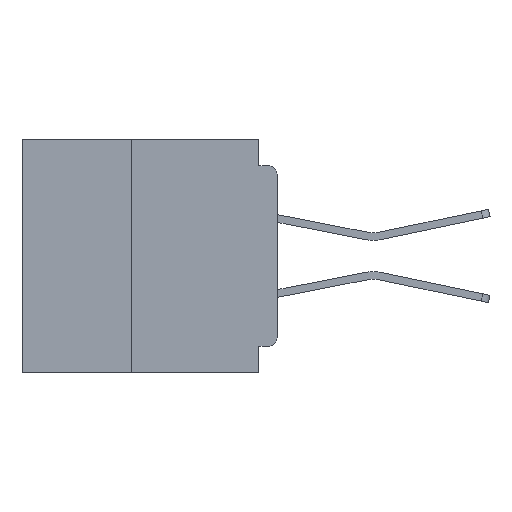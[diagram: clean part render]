
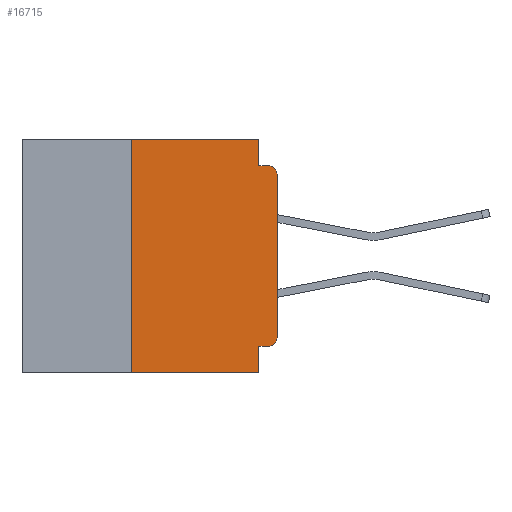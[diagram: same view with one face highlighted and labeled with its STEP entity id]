
A CAD part, left-side view. The second image highlights one B-rep face of the part: STEP entity #16715.
In plain terms, the highlighted planar face has unit normal (-1, 0, 0).
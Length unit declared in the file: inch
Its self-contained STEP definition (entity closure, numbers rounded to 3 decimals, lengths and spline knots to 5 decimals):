
#3455 = CARTESIAN_POINT ( 'NONE',  ( 0., 0., 0. ) ) ;
#4872 = CARTESIAN_POINT ( 'NONE',  ( 0., 0.015, -0.355 ) ) ;
#5386 = DIRECTION ( 'NONE',  ( 0., -1., 0. ) ) ;
#5834 = LINE ( 'NONE', #49728, #11250 ) ;
#6567 = CARTESIAN_POINT ( 'NONE',  ( 0., 0.437, -0.4 ) ) ;
#8471 = DIRECTION ( 'NONE',  ( 0., 0., 1. ) ) ;
#9504 = DIRECTION ( 'NONE',  ( -1., 0., 0. ) ) ;
#9772 = CARTESIAN_POINT ( 'NONE',  ( 0., 0.031, -0.355 ) ) ;
#10374 = EDGE_CURVE ( 'NONE', #25552, #42481, #11845, .T. ) ;
#10798 = DIRECTION ( 'NONE',  ( 0., -1., 0. ) ) ;
#11157 = DIRECTION ( 'NONE',  ( -1., 0., 0. ) ) ;
#11250 = VECTOR ( 'NONE', #5386, 39.37008 ) ;
#11527 = CARTESIAN_POINT ( 'NONE',  ( 0., 0.015, -0.045 ) ) ;
#11551 = DIRECTION ( 'NONE',  ( 0., -1., 0. ) ) ;
#11845 = LINE ( 'NONE', #53822, #62756 ) ;
#13513 = EDGE_CURVE ( 'NONE', #52806, #45331, #13784, .T. ) ;
#13784 = LINE ( 'NONE', #21870, #38605 ) ;
#14184 = LINE ( 'NONE', #3455, #48982 ) ;
#16715 = ADVANCED_FACE ( 'NONE', ( #23453 ), #50948, .F. ) ;
#17158 = CARTESIAN_POINT ( 'NONE',  ( 0., 0.25, 0. ) ) ;
#18208 = CARTESIAN_POINT ( 'NONE',  ( 0., 0.25, -0.4 ) ) ;
#18677 = VERTEX_POINT ( 'NONE', #47923 ) ;
#18728 = LINE ( 'NONE', #40527, #33499 ) ;
#19309 = LINE ( 'NONE', #6567, #44117 ) ;
#19491 = VERTEX_POINT ( 'NONE', #59799 ) ;
#19606 = ORIENTED_EDGE ( 'NONE', *, *, #21280, .F. ) ;
#21280 = EDGE_CURVE ( 'NONE', #45331, #45903, #18728, .T. ) ;
#21620 = AXIS2_PLACEMENT_3D ( 'NONE', #46044, #55880, #26408 ) ;
#21870 = CARTESIAN_POINT ( 'NONE',  ( 0., 0.031, 0. ) ) ;
#23093 = CARTESIAN_POINT ( 'NONE',  ( 0., 0.031, -0.4 ) ) ;
#23453 = FACE_OUTER_BOUND ( 'NONE', #51511, .T. ) ;
#23749 = ORIENTED_EDGE ( 'NONE', *, *, #13513, .F. ) ;
#25552 = VERTEX_POINT ( 'NONE', #4872 ) ;
#25715 = ORIENTED_EDGE ( 'NONE', *, *, #50048, .T. ) ;
#26408 = DIRECTION ( 'NONE',  ( 0., 0., -1. ) ) ;
#27443 = EDGE_CURVE ( 'NONE', #25552, #18677, #63389, .T. ) ;
#29066 = VERTEX_POINT ( 'NONE', #47183 ) ;
#29164 = EDGE_CURVE ( 'NONE', #29066, #30611, #31685, .T. ) ;
#30611 = VERTEX_POINT ( 'NONE', #17158 ) ;
#31685 = LINE ( 'NONE', #18208, #41741 ) ;
#31871 = DIRECTION ( 'NONE',  ( 0., 0., -1. ) ) ;
#33196 = DIRECTION ( 'NONE',  ( 0., 0., 1. ) ) ;
#33471 = VERTEX_POINT ( 'NONE', #23093 ) ;
#33499 = VECTOR ( 'NONE', #10798, 39.37008 ) ;
#33875 = EDGE_CURVE ( 'NONE', #29066, #33471, #19309, .T. ) ;
#35466 = VECTOR ( 'NONE', #45686, 39.37008 ) ;
#36401 = ORIENTED_EDGE ( 'NONE', *, *, #47522, .F. ) ;
#38605 = VECTOR ( 'NONE', #31871, 39.37008 ) ;
#39180 = ORIENTED_EDGE ( 'NONE', *, *, #46411, .F. ) ;
#39201 = CARTESIAN_POINT ( 'NONE',  ( 0., 0.015, -0.34 ) ) ;
#40527 = CARTESIAN_POINT ( 'NONE',  ( 0., 0., -0.045 ) ) ;
#40738 = CARTESIAN_POINT ( 'NONE',  ( 0., 0.031, -0.4 ) ) ;
#40873 = CARTESIAN_POINT ( 'NONE',  ( 0., 0.015, -0.06 ) ) ;
#41687 = LINE ( 'NONE', #40738, #35466 ) ;
#41741 = VECTOR ( 'NONE', #33196, 39.37008 ) ;
#42357 = ORIENTED_EDGE ( 'NONE', *, *, #29164, .F. ) ;
#42481 = VERTEX_POINT ( 'NONE', #9772 ) ;
#44117 = VECTOR ( 'NONE', #11551, 39.37008 ) ;
#44195 = DIRECTION ( 'NONE',  ( 0., 0., -1. ) ) ;
#44206 = DIRECTION ( 'NONE',  ( 0., 1., 0. ) ) ;
#45331 = VERTEX_POINT ( 'NONE', #56497 ) ;
#45686 = DIRECTION ( 'NONE',  ( 0., 0., -1. ) ) ;
#45816 = DIRECTION ( 'NONE',  ( 0., 0., -1. ) ) ;
#45903 = VERTEX_POINT ( 'NONE', #11527 ) ;
#46044 = CARTESIAN_POINT ( 'NONE',  ( 0., 0.437, 0. ) ) ;
#46411 = EDGE_CURVE ( 'NONE', #42481, #33471, #41687, .T. ) ;
#47183 = CARTESIAN_POINT ( 'NONE',  ( 0., 0.25, -0.4 ) ) ;
#47522 = EDGE_CURVE ( 'NONE', #30611, #52806, #5834, .T. ) ;
#47923 = CARTESIAN_POINT ( 'NONE',  ( 0., 0., -0.34 ) ) ;
#48228 = CARTESIAN_POINT ( 'NONE',  ( 0., 0.031, 0. ) ) ;
#48982 = VECTOR ( 'NONE', #8471, 39.37008 ) ;
#49112 = ORIENTED_EDGE ( 'NONE', *, *, #27443, .T. ) ;
#49728 = CARTESIAN_POINT ( 'NONE',  ( 0., 0.437, 0. ) ) ;
#50048 = EDGE_CURVE ( 'NONE', #19491, #45903, #63591, .T. ) ;
#50948 = PLANE ( 'NONE',  #21620 ) ;
#51511 = EDGE_LOOP ( 'NONE', ( #56325, #25715, #19606, #23749, #36401, #42357, #53467, #39180, #52577, #49112 ) ) ;
#52577 = ORIENTED_EDGE ( 'NONE', *, *, #10374, .F. ) ;
#52806 = VERTEX_POINT ( 'NONE', #48228 ) ;
#53467 = ORIENTED_EDGE ( 'NONE', *, *, #33875, .T. ) ;
#53822 = CARTESIAN_POINT ( 'NONE',  ( 0., 0., -0.355 ) ) ;
#55880 = DIRECTION ( 'NONE',  ( 1., 0., 0. ) ) ;
#56325 = ORIENTED_EDGE ( 'NONE', *, *, #62300, .T. ) ;
#56497 = CARTESIAN_POINT ( 'NONE',  ( 0., 0.031, -0.045 ) ) ;
#57014 = AXIS2_PLACEMENT_3D ( 'NONE', #40873, #11157, #45816 ) ;
#59799 = CARTESIAN_POINT ( 'NONE',  ( 0., 0., -0.06 ) ) ;
#61210 = AXIS2_PLACEMENT_3D ( 'NONE', #39201, #9504, #44195 ) ;
#62300 = EDGE_CURVE ( 'NONE', #18677, #19491, #14184, .T. ) ;
#62756 = VECTOR ( 'NONE', #44206, 39.37008 ) ;
#63389 = CIRCLE ( 'NONE', #61210, 0.015 ) ;
#63591 = CIRCLE ( 'NONE', #57014, 0.015 ) ;
